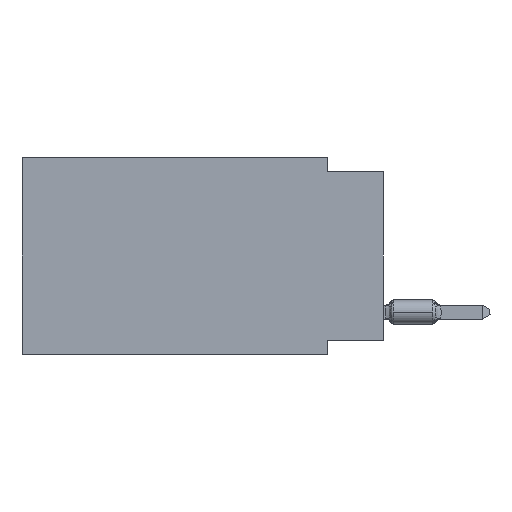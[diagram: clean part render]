
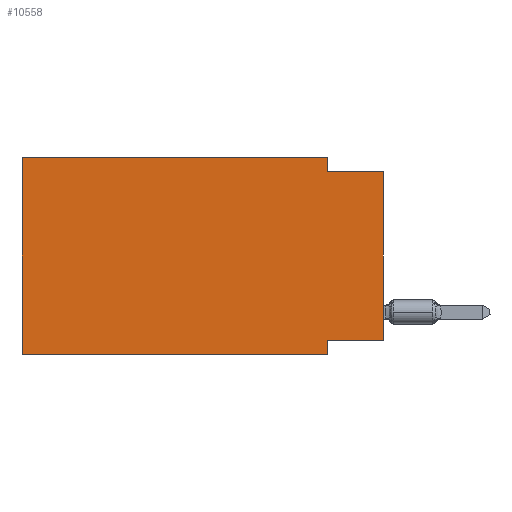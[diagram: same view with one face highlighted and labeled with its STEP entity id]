
A CAD part, left-side view. The second image highlights one B-rep face of the part: STEP entity #10558.
In plain terms, the highlighted planar face has unit normal (-1, 0, 0).
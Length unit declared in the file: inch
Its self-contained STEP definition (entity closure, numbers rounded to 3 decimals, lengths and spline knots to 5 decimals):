
#442 = EDGE_CURVE ( 'NONE', #38406, #43940, #6940, .T. ) ;
#2165 = FACE_OUTER_BOUND ( 'NONE', #47712, .T. ) ;
#3644 = ORIENTED_EDGE ( 'NONE', *, *, #44814, .F. ) ;
#5155 = CARTESIAN_POINT ( 'NONE',  ( 0., 0.1, 0. ) ) ;
#5503 = LINE ( 'NONE', #47149, #5997 ) ;
#5520 = CARTESIAN_POINT ( 'NONE',  ( 0., 0.1, -0.35 ) ) ;
#5913 = VERTEX_POINT ( 'NONE', #20467 ) ;
#5997 = VECTOR ( 'NONE', #40209, 39.37008 ) ;
#6940 = LINE ( 'NONE', #7205, #12766 ) ;
#7205 = CARTESIAN_POINT ( 'NONE',  ( 0., 0., 0. ) ) ;
#8966 = LINE ( 'NONE', #38962, #16406 ) ;
#9397 = VECTOR ( 'NONE', #9422, 39.37008 ) ;
#9422 = DIRECTION ( 'NONE',  ( 0., -1., 0. ) ) ;
#10558 = ADVANCED_FACE ( 'NONE', ( #2165 ), #17575, .F. ) ;
#10872 = EDGE_CURVE ( 'NONE', #5913, #31411, #13067, .T. ) ;
#11667 = ORIENTED_EDGE ( 'NONE', *, *, #442, .T. ) ;
#12177 = CARTESIAN_POINT ( 'NONE',  ( 0., 0., -0.325 ) ) ;
#12766 = VECTOR ( 'NONE', #37218, 39.37008 ) ;
#13067 = LINE ( 'NONE', #20472, #47085 ) ;
#13426 = ORIENTED_EDGE ( 'NONE', *, *, #27404, .T. ) ;
#13837 = CARTESIAN_POINT ( 'NONE',  ( 0., 0.1, -0.025 ) ) ;
#13888 = CARTESIAN_POINT ( 'NONE',  ( 0., 0.645, 0. ) ) ;
#15899 = DIRECTION ( 'NONE',  ( 0., 1., 0. ) ) ;
#16406 = VECTOR ( 'NONE', #33825, 39.37008 ) ;
#16620 = LINE ( 'NONE', #12177, #29291 ) ;
#17068 = DIRECTION ( 'NONE',  ( 0., 0., -1. ) ) ;
#17157 = ORIENTED_EDGE ( 'NONE', *, *, #47595, .F. ) ;
#17290 = VECTOR ( 'NONE', #17068, 39.37008 ) ;
#17575 = PLANE ( 'NONE',  #25013 ) ;
#17603 = LINE ( 'NONE', #13888, #9397 ) ;
#19069 = EDGE_CURVE ( 'NONE', #31411, #38484, #17603, .T. ) ;
#20467 = CARTESIAN_POINT ( 'NONE',  ( 0., 0.645, -0.35 ) ) ;
#20472 = CARTESIAN_POINT ( 'NONE',  ( 0., 0.645, 0. ) ) ;
#20532 = LINE ( 'NONE', #5155, #17290 ) ;
#21023 = DIRECTION ( 'NONE',  ( 0., 0., -1. ) ) ;
#22093 = CARTESIAN_POINT ( 'NONE',  ( 0., 0.645, -0.35 ) ) ;
#23438 = CARTESIAN_POINT ( 'NONE',  ( 0., 0., -0.025 ) ) ;
#25013 = AXIS2_PLACEMENT_3D ( 'NONE', #31943, #44085, #21023 ) ;
#25091 = CARTESIAN_POINT ( 'NONE',  ( 0., 0.1, -0.325 ) ) ;
#27133 = ORIENTED_EDGE ( 'NONE', *, *, #30111, .F. ) ;
#27404 = EDGE_CURVE ( 'NONE', #5913, #35067, #34650, .T. ) ;
#27737 = ORIENTED_EDGE ( 'NONE', *, *, #10872, .F. ) ;
#27759 = VERTEX_POINT ( 'NONE', #13837 ) ;
#27914 = DIRECTION ( 'NONE',  ( 0., 0., 1. ) ) ;
#29291 = VECTOR ( 'NONE', #15899, 39.37008 ) ;
#30111 = EDGE_CURVE ( 'NONE', #38406, #46109, #16620, .T. ) ;
#30673 = DIRECTION ( 'NONE',  ( 0., -1., 0. ) ) ;
#31411 = VERTEX_POINT ( 'NONE', #33455 ) ;
#31943 = CARTESIAN_POINT ( 'NONE',  ( 0., 0.645, 0. ) ) ;
#33455 = CARTESIAN_POINT ( 'NONE',  ( 0., 0.645, 0. ) ) ;
#33825 = DIRECTION ( 'NONE',  ( 0., 0., -1. ) ) ;
#34650 = LINE ( 'NONE', #22093, #46640 ) ;
#34787 = CARTESIAN_POINT ( 'NONE',  ( 0., 0., -0.325 ) ) ;
#35067 = VERTEX_POINT ( 'NONE', #5520 ) ;
#35420 = ORIENTED_EDGE ( 'NONE', *, *, #19069, .F. ) ;
#37218 = DIRECTION ( 'NONE',  ( 0., 0., 1. ) ) ;
#38406 = VERTEX_POINT ( 'NONE', #34787 ) ;
#38484 = VERTEX_POINT ( 'NONE', #42980 ) ;
#38962 = CARTESIAN_POINT ( 'NONE',  ( 0., 0.1, -0.35 ) ) ;
#40209 = DIRECTION ( 'NONE',  ( 0., -1., 0. ) ) ;
#42053 = ORIENTED_EDGE ( 'NONE', *, *, #49007, .F. ) ;
#42980 = CARTESIAN_POINT ( 'NONE',  ( 0., 0.1, 0. ) ) ;
#43940 = VERTEX_POINT ( 'NONE', #23438 ) ;
#44085 = DIRECTION ( 'NONE',  ( 1., 0., 0. ) ) ;
#44814 = EDGE_CURVE ( 'NONE', #27759, #43940, #5503, .T. ) ;
#46109 = VERTEX_POINT ( 'NONE', #25091 ) ;
#46640 = VECTOR ( 'NONE', #30673, 39.37008 ) ;
#47085 = VECTOR ( 'NONE', #27914, 39.37008 ) ;
#47149 = CARTESIAN_POINT ( 'NONE',  ( 0., 0., -0.025 ) ) ;
#47595 = EDGE_CURVE ( 'NONE', #46109, #35067, #8966, .T. ) ;
#47712 = EDGE_LOOP ( 'NONE', ( #11667, #3644, #42053, #35420, #27737, #13426, #17157, #27133 ) ) ;
#49007 = EDGE_CURVE ( 'NONE', #38484, #27759, #20532, .T. ) ;
